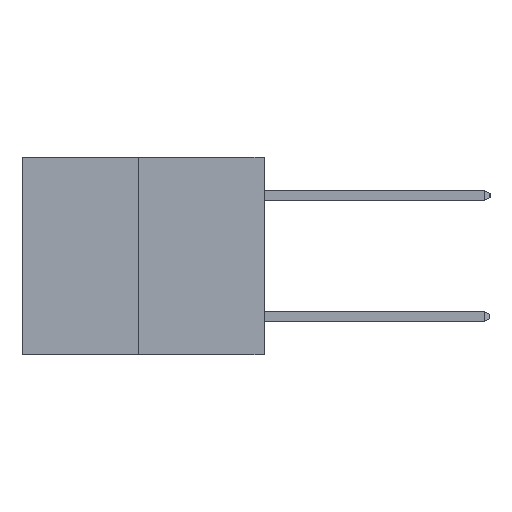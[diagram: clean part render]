
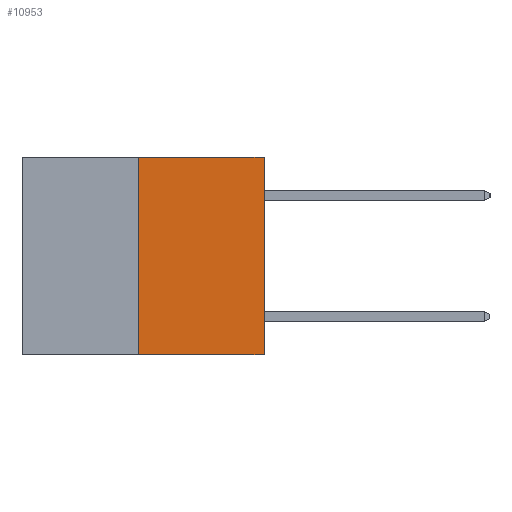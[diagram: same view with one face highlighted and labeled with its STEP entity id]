
A CAD part, left-side view. The second image highlights one B-rep face of the part: STEP entity #10953.
In plain terms, the highlighted planar face has unit normal (-1, 0, 0).
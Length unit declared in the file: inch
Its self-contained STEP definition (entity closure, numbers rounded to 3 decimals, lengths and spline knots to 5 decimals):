
#408 = ORIENTED_EDGE ( 'NONE', *, *, #3982, .F. ) ;
#1281 = EDGE_LOOP ( 'NONE', ( #408, #2086, #11318, #2150 ) ) ;
#1657 = EDGE_CURVE ( 'NONE', #7817, #4800, #6980, .T. ) ;
#2070 = CARTESIAN_POINT ( 'NONE',  ( 0., 0.6, -0.49 ) ) ;
#2086 = ORIENTED_EDGE ( 'NONE', *, *, #1657, .T. ) ;
#2150 = ORIENTED_EDGE ( 'NONE', *, *, #8233, .F. ) ;
#3982 = EDGE_CURVE ( 'NONE', #7817, #7287, #7151, .T. ) ;
#4035 = EDGE_CURVE ( 'NONE', #4800, #7005, #9503, .T. ) ;
#4311 = DIRECTION ( 'NONE',  ( 0., -1., 0. ) ) ;
#4369 = DIRECTION ( 'NONE',  ( 0., 0., -1. ) ) ;
#4495 = DIRECTION ( 'NONE',  ( 1., 0., 0. ) ) ;
#4758 = AXIS2_PLACEMENT_3D ( 'NONE', #6439, #4495, #4369 ) ;
#4800 = VERTEX_POINT ( 'NONE', #9380 ) ;
#5403 = VECTOR ( 'NONE', #8072, 39.37008 ) ;
#5859 = DIRECTION ( 'NONE',  ( 0., 0., 1. ) ) ;
#6439 = CARTESIAN_POINT ( 'NONE',  ( 0., 0.6, 0. ) ) ;
#6980 = LINE ( 'NONE', #2070, #5403 ) ;
#7005 = VERTEX_POINT ( 'NONE', #11985 ) ;
#7078 = VECTOR ( 'NONE', #4311, 39.37008 ) ;
#7151 = LINE ( 'NONE', #9919, #11501 ) ;
#7287 = VERTEX_POINT ( 'NONE', #8686 ) ;
#7388 = LINE ( 'NONE', #8283, #7078 ) ;
#7817 = VERTEX_POINT ( 'NONE', #8418 ) ;
#8072 = DIRECTION ( 'NONE',  ( 0., -1., 0. ) ) ;
#8135 = DIRECTION ( 'NONE',  ( 0., 0., 1. ) ) ;
#8233 = EDGE_CURVE ( 'NONE', #7287, #7005, #7388, .T. ) ;
#8283 = CARTESIAN_POINT ( 'NONE',  ( 0., 0.6, 0. ) ) ;
#8418 = CARTESIAN_POINT ( 'NONE',  ( 0., 0.312, -0.49 ) ) ;
#8467 = PLANE ( 'NONE',  #4758 ) ;
#8686 = CARTESIAN_POINT ( 'NONE',  ( 0., 0.312, 0. ) ) ;
#9380 = CARTESIAN_POINT ( 'NONE',  ( 0., 0., -0.49 ) ) ;
#9503 = LINE ( 'NONE', #10132, #12582 ) ;
#9919 = CARTESIAN_POINT ( 'NONE',  ( 0., 0.312, -0.49 ) ) ;
#10132 = CARTESIAN_POINT ( 'NONE',  ( 0., 0., 0. ) ) ;
#10953 = ADVANCED_FACE ( 'NONE', ( #11427 ), #8467, .F. ) ;
#11318 = ORIENTED_EDGE ( 'NONE', *, *, #4035, .T. ) ;
#11427 = FACE_OUTER_BOUND ( 'NONE', #1281, .T. ) ;
#11501 = VECTOR ( 'NONE', #5859, 39.37008 ) ;
#11985 = CARTESIAN_POINT ( 'NONE',  ( 0., 0., 0. ) ) ;
#12582 = VECTOR ( 'NONE', #8135, 39.37008 ) ;
